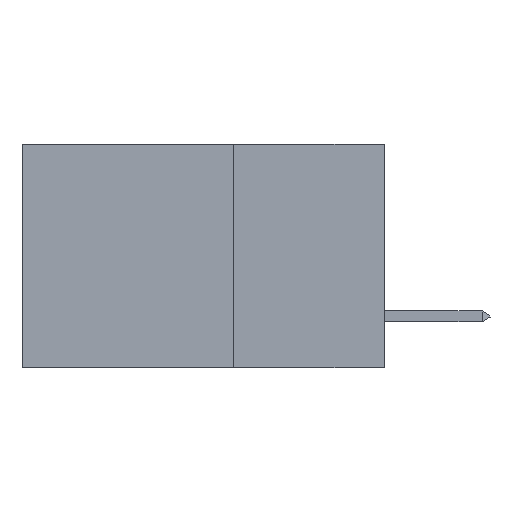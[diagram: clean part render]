
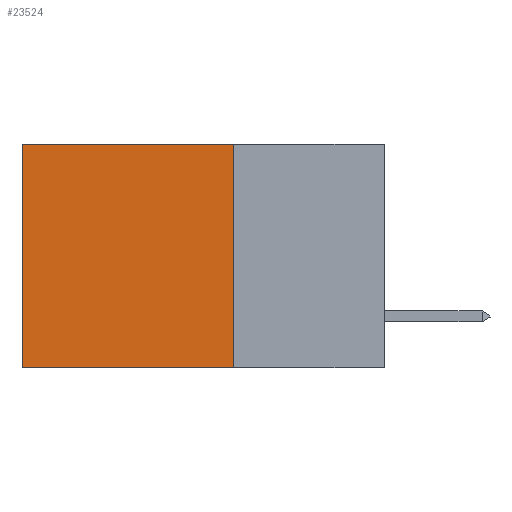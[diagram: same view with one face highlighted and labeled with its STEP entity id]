
A CAD part, left-side view. The second image highlights one B-rep face of the part: STEP entity #23524.
In plain terms, the highlighted planar face has unit normal (-1, 0, 0).
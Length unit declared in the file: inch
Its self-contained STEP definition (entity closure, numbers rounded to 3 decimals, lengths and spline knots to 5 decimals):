
#278 = VERTEX_POINT ( 'NONE', #2055 ) ;
#813 = AXIS2_PLACEMENT_3D ( 'NONE', #26551, #15565, #9658 ) ;
#1503 = EDGE_CURVE ( 'NONE', #24187, #15477, #27031, .T. ) ;
#1520 = EDGE_CURVE ( 'NONE', #11863, #24187, #22092, .T. ) ;
#1908 = DIRECTION ( 'NONE',  ( 0., 1., 0. ) ) ;
#2055 = CARTESIAN_POINT ( 'NONE',  ( 0.2875, 0.6, 0. ) ) ;
#2881 = CARTESIAN_POINT ( 'NONE',  ( 0.2875, 0.25, 0. ) ) ;
#3596 = ORIENTED_EDGE ( 'NONE', *, *, #26706, .T. ) ;
#6679 = LINE ( 'NONE', #12155, #27214 ) ;
#6915 = DIRECTION ( 'NONE',  ( 0., 1., 0. ) ) ;
#7883 = ORIENTED_EDGE ( 'NONE', *, *, #1520, .F. ) ;
#9648 = CARTESIAN_POINT ( 'NONE',  ( 0.2875, 0.25, 0. ) ) ;
#9658 = DIRECTION ( 'NONE',  ( 0., 0., -1. ) ) ;
#11863 = VERTEX_POINT ( 'NONE', #9648 ) ;
#12047 = EDGE_CURVE ( 'NONE', #278, #15477, #6679, .T. ) ;
#12155 = CARTESIAN_POINT ( 'NONE',  ( 0.2875, 0.6, 0. ) ) ;
#13075 = VECTOR ( 'NONE', #6915, 39.37008 ) ;
#14440 = VECTOR ( 'NONE', #1908, 39.37008 ) ;
#15477 = VERTEX_POINT ( 'NONE', #19666 ) ;
#15565 = DIRECTION ( 'NONE',  ( 1., 0., 0. ) ) ;
#16468 = DIRECTION ( 'NONE',  ( 0., 0., -1. ) ) ;
#16833 = ORIENTED_EDGE ( 'NONE', *, *, #1503, .F. ) ;
#17183 = EDGE_LOOP ( 'NONE', ( #22609, #16833, #7883, #3596 ) ) ;
#17715 = LINE ( 'NONE', #2881, #13075 ) ;
#19666 = CARTESIAN_POINT ( 'NONE',  ( 0.2875, 0.6, -0.37 ) ) ;
#19875 = CARTESIAN_POINT ( 'NONE',  ( 0.2875, 0.25, -0.37 ) ) ;
#22092 = LINE ( 'NONE', #26848, #25006 ) ;
#22609 = ORIENTED_EDGE ( 'NONE', *, *, #12047, .T. ) ;
#23067 = CARTESIAN_POINT ( 'NONE',  ( 0.2875, 0.25, -0.37 ) ) ;
#23524 = ADVANCED_FACE ( 'NONE', ( #27145 ), #24152, .F. ) ;
#24152 = PLANE ( 'NONE',  #813 ) ;
#24187 = VERTEX_POINT ( 'NONE', #19875 ) ;
#24895 = DIRECTION ( 'NONE',  ( 0., 0., -1. ) ) ;
#25006 = VECTOR ( 'NONE', #16468, 39.37008 ) ;
#26551 = CARTESIAN_POINT ( 'NONE',  ( 0.2875, 0.25, 0. ) ) ;
#26706 = EDGE_CURVE ( 'NONE', #11863, #278, #17715, .T. ) ;
#26848 = CARTESIAN_POINT ( 'NONE',  ( 0.2875, 0.25, 0. ) ) ;
#27031 = LINE ( 'NONE', #23067, #14440 ) ;
#27145 = FACE_OUTER_BOUND ( 'NONE', #17183, .T. ) ;
#27214 = VECTOR ( 'NONE', #24895, 39.37008 ) ;
